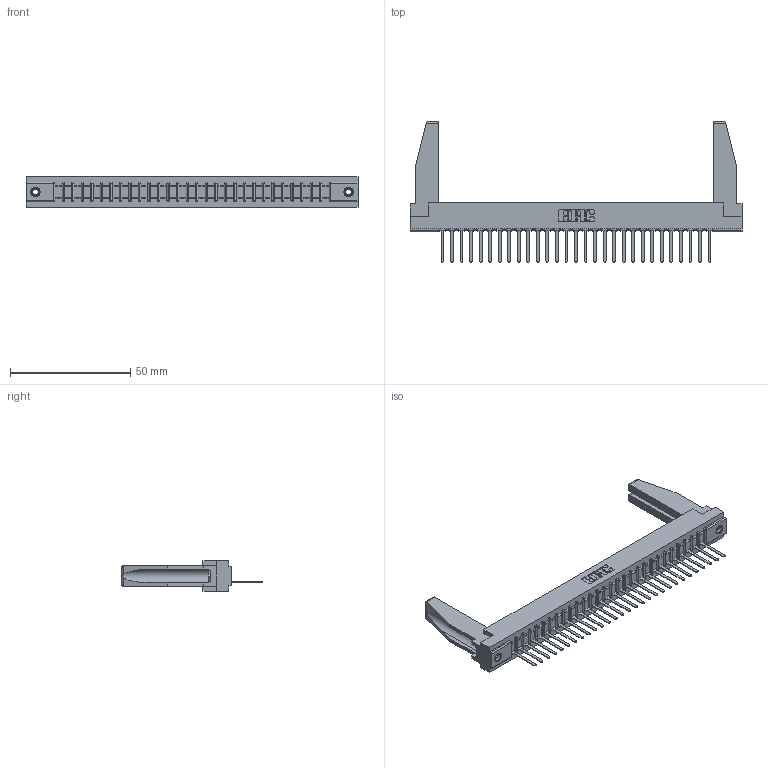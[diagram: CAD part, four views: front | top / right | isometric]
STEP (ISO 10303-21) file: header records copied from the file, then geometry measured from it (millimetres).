
FILE_DESCRIPTION (( 'STEP AP203' ), '1' );
FILE_NAME ('307-029-541-178.STEP', '2019-09-05T03:42:13', ( '' ), ( '' ), 'SwSTEP 2.0', 'SolidWorks 2016', '' );
FILE_SCHEMA (( 'CONFIG_CONTROL_DESIGN' ));
Length unit declared in the file: inch
Products named in the file (5): 307-220-078; 307 Part_.156 Dia Mounting Holes; 307-290-002_541; 345-250-001_345-250-001-102; 307-029-541-178
Assembly tree (34 placements, depth 2):
  307-029-541-178
    307 Part_.156 Dia Mounting Holes
    307-290-002_541  x29
    307-220-078  x2
    345-250-001_345-250-001-102  x2
Bounding box: 137.92 x 58.29 x 12.7 mm (x, y, z)
Volume: 18737.6 mm3; surface area: 22606.3 mm2
Topology: 34 solids, 34 shells, 2424 faces, 7381 edges, 4830 vertices
Faces by surface type: plane 1459, cylinder 889, sphere 60, cone 12, torus 4
Entity records: 29621 total; most frequent: CARTESIAN_POINT 4994, ORIENTED_EDGE 4940, DIRECTION 4814, EDGE_CURVE 2470, LINE 1890, VECTOR 1890, VERTEX_POINT 1600, AXIS2_PLACEMENT_3D 1462
